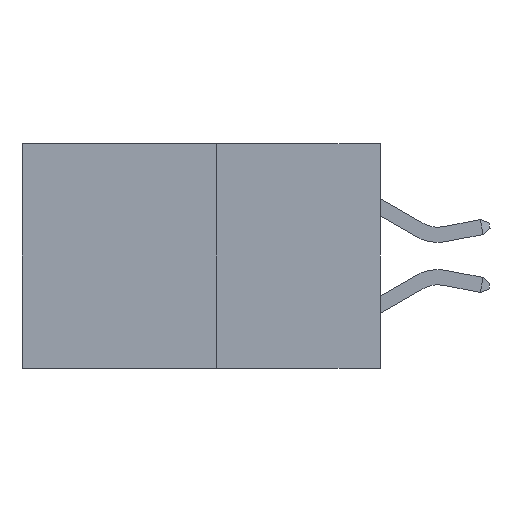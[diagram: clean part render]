
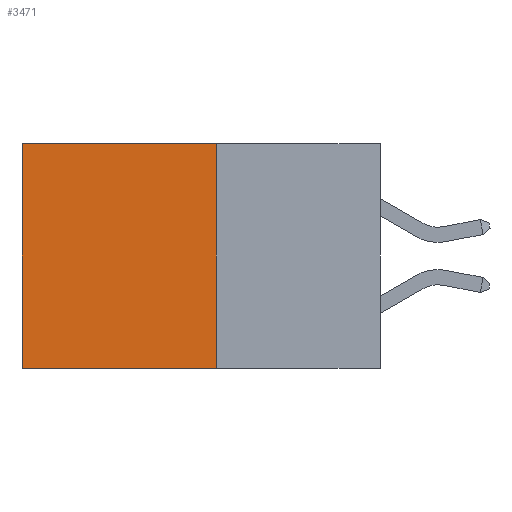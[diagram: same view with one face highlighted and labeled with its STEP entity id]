
A CAD part, left-side view. The second image highlights one B-rep face of the part: STEP entity #3471.
In plain terms, the highlighted planar face has unit normal (-1, 0, 0).
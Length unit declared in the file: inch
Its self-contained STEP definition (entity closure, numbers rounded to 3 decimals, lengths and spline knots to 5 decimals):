
#132 = LINE ( 'NONE', #4522, #8619 ) ;
#977 = VERTEX_POINT ( 'NONE', #9132 ) ;
#1079 = DIRECTION ( 'NONE',  ( 1., 0., 0. ) ) ;
#1278 = ORIENTED_EDGE ( 'NONE', *, *, #3319, .F. ) ;
#1441 = DIRECTION ( 'NONE',  ( 0., 0., -1. ) ) ;
#1480 = PLANE ( 'NONE',  #8161 ) ;
#1819 = CARTESIAN_POINT ( 'NONE',  ( 0.277, 0.27, -0.37 ) ) ;
#1995 = VECTOR ( 'NONE', #9607, 39.37008 ) ;
#2148 = VECTOR ( 'NONE', #4518, 39.37008 ) ;
#2408 = VERTEX_POINT ( 'NONE', #9838 ) ;
#2892 = EDGE_CURVE ( 'NONE', #10005, #2408, #6580, .T. ) ;
#3319 = EDGE_CURVE ( 'NONE', #977, #9254, #132, .T. ) ;
#3471 = ADVANCED_FACE ( 'NONE', ( #7197 ), #1480, .F. ) ;
#3797 = ORIENTED_EDGE ( 'NONE', *, *, #5785, .T. ) ;
#4023 = EDGE_CURVE ( 'NONE', #10005, #977, #8243, .T. ) ;
#4518 = DIRECTION ( 'NONE',  ( 0., 1., 0. ) ) ;
#4522 = CARTESIAN_POINT ( 'NONE',  ( 0.277, 0.27, -0.37 ) ) ;
#4637 = CARTESIAN_POINT ( 'NONE',  ( 0.277, 0.27, 0. ) ) ;
#4887 = DIRECTION ( 'NONE',  ( 0., 0., -1. ) ) ;
#5251 = ORIENTED_EDGE ( 'NONE', *, *, #2892, .T. ) ;
#5296 = CARTESIAN_POINT ( 'NONE',  ( 0.277, 0.59, -0.37 ) ) ;
#5785 = EDGE_CURVE ( 'NONE', #2408, #9254, #8685, .T. ) ;
#6371 = ORIENTED_EDGE ( 'NONE', *, *, #4023, .F. ) ;
#6580 = LINE ( 'NONE', #4637, #2148 ) ;
#7197 = FACE_OUTER_BOUND ( 'NONE', #9637, .T. ) ;
#8082 = CARTESIAN_POINT ( 'NONE',  ( 0.277, 0.59, -0.37 ) ) ;
#8161 = AXIS2_PLACEMENT_3D ( 'NONE', #1819, #1079, #1441 ) ;
#8208 = VECTOR ( 'NONE', #4887, 39.37008 ) ;
#8243 = LINE ( 'NONE', #9818, #1995 ) ;
#8619 = VECTOR ( 'NONE', #9825, 39.37008 ) ;
#8685 = LINE ( 'NONE', #8082, #8208 ) ;
#9132 = CARTESIAN_POINT ( 'NONE',  ( 0.277, 0.27, -0.37 ) ) ;
#9254 = VERTEX_POINT ( 'NONE', #5296 ) ;
#9529 = CARTESIAN_POINT ( 'NONE',  ( 0.277, 0.27, 0. ) ) ;
#9607 = DIRECTION ( 'NONE',  ( 0., 0., -1. ) ) ;
#9637 = EDGE_LOOP ( 'NONE', ( #3797, #1278, #6371, #5251 ) ) ;
#9818 = CARTESIAN_POINT ( 'NONE',  ( 0.277, 0.27, -0.37 ) ) ;
#9825 = DIRECTION ( 'NONE',  ( 0., 1., 0. ) ) ;
#9838 = CARTESIAN_POINT ( 'NONE',  ( 0.277, 0.59, 0. ) ) ;
#10005 = VERTEX_POINT ( 'NONE', #9529 ) ;
